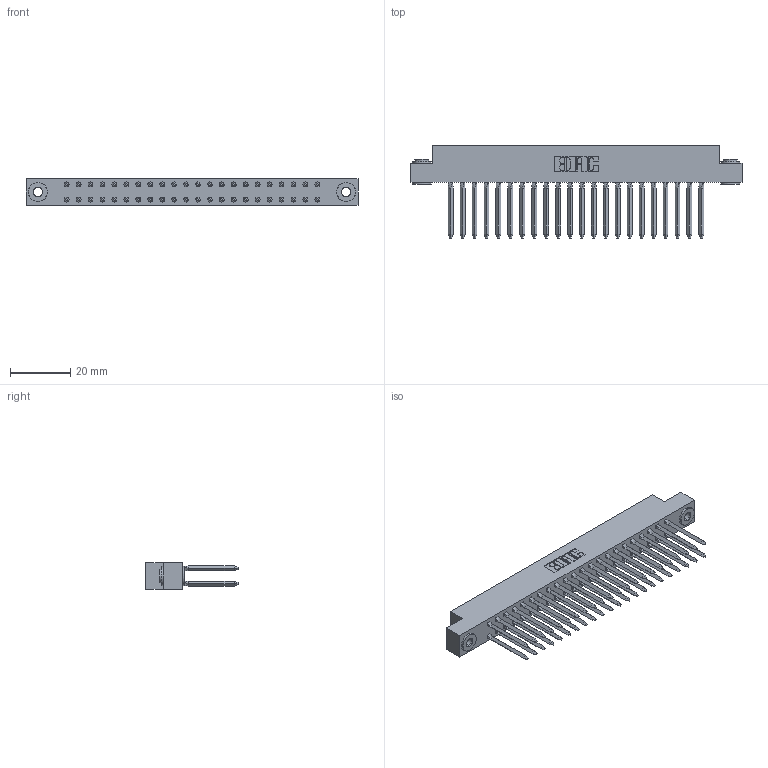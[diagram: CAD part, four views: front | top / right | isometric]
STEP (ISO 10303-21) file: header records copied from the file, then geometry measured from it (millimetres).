
FILE_DESCRIPTION (( 'STEP AP203' ), '1' );
FILE_NAME ('338-044-541-203.STEP', '2020-03-24T18:39:58', ( '' ), ( '' ), 'SwSTEP 2.0', 'SolidWorks 2016', '' );
FILE_SCHEMA (( 'CONFIG_CONTROL_DESIGN' ));
Length unit declared in the file: inch
Products named in the file (4): 338-044-541-203; 345-250-002_345-250-002-102; 338-210-001_338-210-022-004; 338-290-001_541
Assembly tree (47 placements, depth 2):
  338-044-541-203
    338-210-001_338-210-022-004
    338-290-001_541  x44
    345-250-002_345-250-002-102  x2
Bounding box: 110.19 x 30.56 x 8.71 mm (x, y, z)
Volume: 8464.5 mm3; surface area: 15903.7 mm2
Topology: 47 solids, 47 shells, 3094 faces, 8283 edges, 5254 vertices
Faces by surface type: plane 2142, cylinder 768, bspline 176, cone 8
Entity records: 46045 total; most frequent: CARTESIAN_POINT 9101, ORIENTED_EDGE 7632, DIRECTION 7185, EDGE_CURVE 3816, VECTOR 2829, LINE 2829, VERTEX_POINT 2478, AXIS2_PLACEMENT_3D 2178
